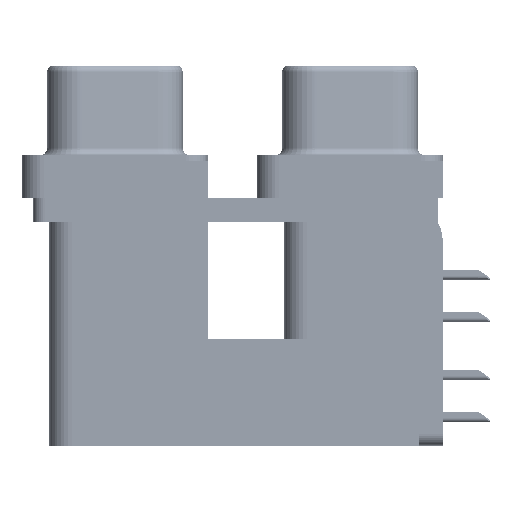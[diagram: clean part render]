
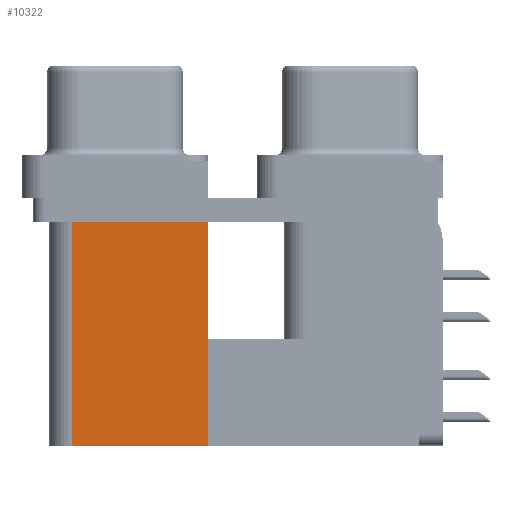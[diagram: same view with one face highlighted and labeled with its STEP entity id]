
A CAD part, left-side view. The second image highlights one B-rep face of the part: STEP entity #10322.
In plain terms, the highlighted planar face has unit normal (-1, 0, 0).
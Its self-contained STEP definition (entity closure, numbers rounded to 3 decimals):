
#514 = EDGE_LOOP ( 'NONE', ( #3917, #8961, #14229, #14811 ) ) ;
#817 = VERTEX_POINT ( 'NONE', #43898 ) ;
#1139 = DIRECTION ( 'NONE',  ( 0., 0., -1. ) ) ;
#3917 = ORIENTED_EDGE ( 'NONE', *, *, #5229, .T. ) ;
#5229 = EDGE_CURVE ( 'NONE', #817, #17446, #40856, .T. ) ;
#5377 = DIRECTION ( 'NONE',  ( 0., 1., 0. ) ) ;
#6256 = EDGE_CURVE ( 'NONE', #12406, #817, #24022, .T. ) ;
#8610 = CARTESIAN_POINT ( 'NONE',  ( 3.79, 9.6, -19.2 ) ) ;
#8961 = ORIENTED_EDGE ( 'NONE', *, *, #41942, .F. ) ;
#10322 = ADVANCED_FACE ( 'NONE', ( #12238 ), #20200, .F. ) ;
#12238 = FACE_OUTER_BOUND ( 'NONE', #514, .T. ) ;
#12406 = VERTEX_POINT ( 'NONE', #26799 ) ;
#14229 = ORIENTED_EDGE ( 'NONE', *, *, #36977, .F. ) ;
#14377 = CARTESIAN_POINT ( 'NONE',  ( 3.79, 18.8, -2.5 ) ) ;
#14811 = ORIENTED_EDGE ( 'NONE', *, *, #6256, .T. ) ;
#17446 = VERTEX_POINT ( 'NONE', #14377 ) ;
#17777 = VECTOR ( 'NONE', #19404, 1000. ) ;
#17881 = VECTOR ( 'NONE', #41028, 1000. ) ;
#19404 = DIRECTION ( 'NONE',  ( 0., 0., 1. ) ) ;
#20200 = PLANE ( 'NONE',  #30198 ) ;
#24022 = LINE ( 'NONE', #38691, #17777 ) ;
#26799 = CARTESIAN_POINT ( 'NONE',  ( 3.79, 9.6, -19.2 ) ) ;
#30198 = AXIS2_PLACEMENT_3D ( 'NONE', #8610, #47715, #1139 ) ;
#33305 = VERTEX_POINT ( 'NONE', #48662 ) ;
#36977 = EDGE_CURVE ( 'NONE', #12406, #33305, #49271, .T. ) ;
#37016 = CARTESIAN_POINT ( 'NONE',  ( 3.79, 9.6, -2.5 ) ) ;
#37024 = VECTOR ( 'NONE', #49178, 1000. ) ;
#37310 = VECTOR ( 'NONE', #5377, 1000. ) ;
#38691 = CARTESIAN_POINT ( 'NONE',  ( 3.79, 9.6, -19.2 ) ) ;
#40856 = LINE ( 'NONE', #37016, #37310 ) ;
#41028 = DIRECTION ( 'NONE',  ( 0., 1., 0. ) ) ;
#41942 = EDGE_CURVE ( 'NONE', #33305, #17446, #41964, .T. ) ;
#41964 = LINE ( 'NONE', #45570, #37024 ) ;
#43898 = CARTESIAN_POINT ( 'NONE',  ( 3.79, 9.6, -2.5 ) ) ;
#45570 = CARTESIAN_POINT ( 'NONE',  ( 3.79, 18.8, -19.2 ) ) ;
#47715 = DIRECTION ( 'NONE',  ( 1., 0., 0. ) ) ;
#48239 = CARTESIAN_POINT ( 'NONE',  ( 3.79, 9.6, -19.2 ) ) ;
#48662 = CARTESIAN_POINT ( 'NONE',  ( 3.79, 18.8, -19.2 ) ) ;
#49178 = DIRECTION ( 'NONE',  ( 0., 0., 1. ) ) ;
#49271 = LINE ( 'NONE', #48239, #17881 ) ;
